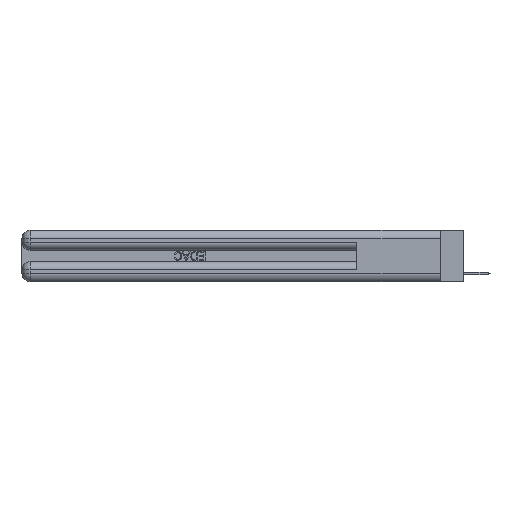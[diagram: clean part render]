
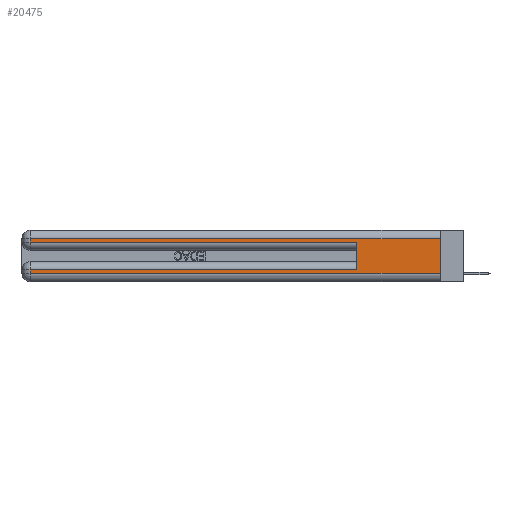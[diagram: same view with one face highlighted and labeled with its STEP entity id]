
A CAD part, left-side view. The second image highlights one B-rep face of the part: STEP entity #20475.
In plain terms, the highlighted planar face has unit normal (-1, 0, 0).
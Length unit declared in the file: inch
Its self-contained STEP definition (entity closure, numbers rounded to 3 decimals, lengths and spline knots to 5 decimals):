
#336 = VERTEX_POINT ( 'NONE', #27947 ) ;
#555 = VECTOR ( 'NONE', #28525, 39.37008 ) ;
#931 = CARTESIAN_POINT ( 'NONE',  ( 0., 0., 0.285 ) ) ;
#1438 = ORIENTED_EDGE ( 'NONE', *, *, #9204, .T. ) ;
#1527 = EDGE_CURVE ( 'NONE', #22381, #16833, #28207, .T. ) ;
#1572 = CARTESIAN_POINT ( 'NONE',  ( 0., 0., 0.37 ) ) ;
#1833 = VECTOR ( 'NONE', #14370, 39.37008 ) ;
#1914 = CARTESIAN_POINT ( 'NONE',  ( 0., 2.94, 0.085 ) ) ;
#2323 = VERTEX_POINT ( 'NONE', #17332 ) ;
#3921 = DIRECTION ( 'NONE',  ( 0., 0., -1. ) ) ;
#4215 = CARTESIAN_POINT ( 'NONE',  ( 0., 2.94, 0.37 ) ) ;
#4902 = VECTOR ( 'NONE', #3921, 39.37008 ) ;
#5744 = LINE ( 'NONE', #931, #20789 ) ;
#6269 = CARTESIAN_POINT ( 'NONE',  ( 0., 0., 0.37 ) ) ;
#6390 = FACE_OUTER_BOUND ( 'NONE', #21308, .T. ) ;
#6513 = EDGE_CURVE ( 'NONE', #22381, #17429, #17353, .T. ) ;
#7575 = ORIENTED_EDGE ( 'NONE', *, *, #21309, .F. ) ;
#7817 = CARTESIAN_POINT ( 'NONE',  ( 0., 0., 0.06 ) ) ;
#8316 = VERTEX_POINT ( 'NONE', #11146 ) ;
#9204 = EDGE_CURVE ( 'NONE', #2323, #16833, #5744, .T. ) ;
#9285 = CARTESIAN_POINT ( 'NONE',  ( 0., 0., 0.31 ) ) ;
#10194 = EDGE_CURVE ( 'NONE', #15313, #336, #18141, .T. ) ;
#11146 = CARTESIAN_POINT ( 'NONE',  ( 0., 0., 0.06 ) ) ;
#11604 = EDGE_CURVE ( 'NONE', #336, #2323, #24320, .T. ) ;
#12093 = CARTESIAN_POINT ( 'NONE',  ( 0., 0.6, 0.285 ) ) ;
#12358 = ORIENTED_EDGE ( 'NONE', *, *, #11604, .T. ) ;
#12498 = ORIENTED_EDGE ( 'NONE', *, *, #21052, .T. ) ;
#14103 = CARTESIAN_POINT ( 'NONE',  ( 0., 2.94, 0.06 ) ) ;
#14370 = DIRECTION ( 'NONE',  ( 0., 0., 1. ) ) ;
#14715 = DIRECTION ( 'NONE',  ( 0., -1., 0. ) ) ;
#15313 = VERTEX_POINT ( 'NONE', #19380 ) ;
#15724 = VECTOR ( 'NONE', #24490, 39.37008 ) ;
#16833 = VERTEX_POINT ( 'NONE', #12093 ) ;
#17332 = CARTESIAN_POINT ( 'NONE',  ( 0., 2.94, 0.285 ) ) ;
#17353 = LINE ( 'NONE', #22187, #555 ) ;
#17429 = VERTEX_POINT ( 'NONE', #1914 ) ;
#17562 = PLANE ( 'NONE',  #19870 ) ;
#17592 = VECTOR ( 'NONE', #19909, 39.37008 ) ;
#17623 = ORIENTED_EDGE ( 'NONE', *, *, #22877, .T. ) ;
#18141 = LINE ( 'NONE', #9285, #28391 ) ;
#19067 = CARTESIAN_POINT ( 'NONE',  ( 0., 0.6, 0.145 ) ) ;
#19380 = CARTESIAN_POINT ( 'NONE',  ( 0., 0., 0.31 ) ) ;
#19503 = LINE ( 'NONE', #22306, #15724 ) ;
#19766 = LINE ( 'NONE', #6269, #17592 ) ;
#19870 = AXIS2_PLACEMENT_3D ( 'NONE', #1572, #23725, #26545 ) ;
#19909 = DIRECTION ( 'NONE',  ( 0., 0., -1. ) ) ;
#20475 = ADVANCED_FACE ( 'NONE', ( #6390 ), #17562, .F. ) ;
#20789 = VECTOR ( 'NONE', #14715, 39.37008 ) ;
#20908 = VECTOR ( 'NONE', #25774, 39.37008 ) ;
#21052 = EDGE_CURVE ( 'NONE', #17429, #27431, #19503, .T. ) ;
#21308 = EDGE_LOOP ( 'NONE', ( #7575, #21568, #12358, #1438, #28962, #27339, #12498, #17623 ) ) ;
#21309 = EDGE_CURVE ( 'NONE', #15313, #8316, #19766, .T. ) ;
#21352 = CARTESIAN_POINT ( 'NONE',  ( 0., 0.6, 0.085 ) ) ;
#21568 = ORIENTED_EDGE ( 'NONE', *, *, #10194, .T. ) ;
#22187 = CARTESIAN_POINT ( 'NONE',  ( 0., 0., 0.085 ) ) ;
#22306 = CARTESIAN_POINT ( 'NONE',  ( 0., 2.94, 0.37 ) ) ;
#22381 = VERTEX_POINT ( 'NONE', #21352 ) ;
#22877 = EDGE_CURVE ( 'NONE', #27431, #8316, #28274, .T. ) ;
#23725 = DIRECTION ( 'NONE',  ( 1., 0., 0. ) ) ;
#24320 = LINE ( 'NONE', #4215, #4902 ) ;
#24490 = DIRECTION ( 'NONE',  ( 0., 0., -1. ) ) ;
#25774 = DIRECTION ( 'NONE',  ( 0., -1., 0. ) ) ;
#26545 = DIRECTION ( 'NONE',  ( 0., 0., -1. ) ) ;
#27339 = ORIENTED_EDGE ( 'NONE', *, *, #6513, .T. ) ;
#27431 = VERTEX_POINT ( 'NONE', #14103 ) ;
#27947 = CARTESIAN_POINT ( 'NONE',  ( 0., 2.94, 0.31 ) ) ;
#28207 = LINE ( 'NONE', #19067, #1833 ) ;
#28274 = LINE ( 'NONE', #7817, #20908 ) ;
#28391 = VECTOR ( 'NONE', #29001, 39.37008 ) ;
#28525 = DIRECTION ( 'NONE',  ( 0., 1., 0. ) ) ;
#28962 = ORIENTED_EDGE ( 'NONE', *, *, #1527, .F. ) ;
#29001 = DIRECTION ( 'NONE',  ( 0., 1., 0. ) ) ;
